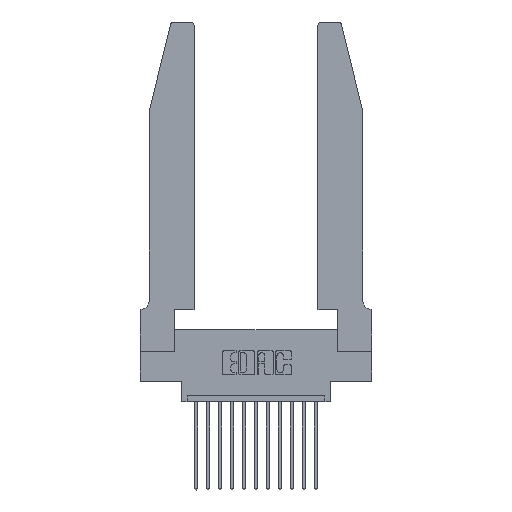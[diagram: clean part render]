
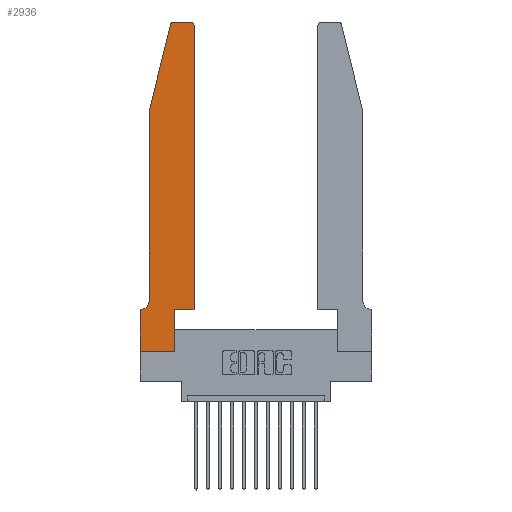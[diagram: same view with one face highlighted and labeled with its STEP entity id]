
A CAD part, top view. The second image highlights one B-rep face of the part: STEP entity #2936.
In plain terms, the highlighted planar face has unit normal (0, 0, 1).
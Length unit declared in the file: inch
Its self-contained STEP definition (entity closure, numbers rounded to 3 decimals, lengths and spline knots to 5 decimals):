
#218 = CARTESIAN_POINT ( 'NONE',  ( 0.4505, 0.35, 0.37 ) ) ;
#524 = VECTOR ( 'NONE', #14686, 39.37008 ) ;
#703 = EDGE_CURVE ( 'NONE', #8851, #9244, #15966, .T. ) ;
#982 = CIRCLE ( 'NONE', #16552, 0.03 ) ;
#1144 = DIRECTION ( 'NONE',  ( 0., 0., -1. ) ) ;
#1153 = VERTEX_POINT ( 'NONE', #10646 ) ;
#1283 = ORIENTED_EDGE ( 'NONE', *, *, #15744, .T. ) ;
#1288 = VERTEX_POINT ( 'NONE', #3385 ) ;
#1454 = VECTOR ( 'NONE', #7306, 39.37008 ) ;
#1493 = AXIS2_PLACEMENT_3D ( 'NONE', #8289, #6906, #9633 ) ;
#1784 = LINE ( 'NONE', #15806, #14376 ) ;
#2375 = DIRECTION ( 'NONE',  ( 0., 0., 1. ) ) ;
#2543 = DIRECTION ( 'NONE',  ( 1., 0., 0. ) ) ;
#2564 = DIRECTION ( 'NONE',  ( -1., 0., 0. ) ) ;
#2749 = CARTESIAN_POINT ( 'NONE',  ( 0., 0., 0.37 ) ) ;
#2924 = ORIENTED_EDGE ( 'NONE', *, *, #3861, .T. ) ;
#2930 = LINE ( 'NONE', #4399, #8323 ) ;
#2936 = ADVANCED_FACE ( 'NONE', ( #8932 ), #13617, .T. ) ;
#3160 = CARTESIAN_POINT ( 'NONE',  ( 0.0055, 0.42, 0.37 ) ) ;
#3186 = LINE ( 'NONE', #16306, #5674 ) ;
#3196 = CARTESIAN_POINT ( 'NONE',  ( 0.25487, 2.72718, 0.37 ) ) ;
#3385 = CARTESIAN_POINT ( 'NONE',  ( 0.4505, 2.72, 0.37 ) ) ;
#3501 = DIRECTION ( 'NONE',  ( 1., 0., 0. ) ) ;
#3754 = EDGE_CURVE ( 'NONE', #15137, #3875, #2930, .T. ) ;
#3861 = EDGE_CURVE ( 'NONE', #1153, #13302, #14398, .T. ) ;
#3875 = VERTEX_POINT ( 'NONE', #11994 ) ;
#4043 = CARTESIAN_POINT ( 'NONE',  ( 0.2865, 0.35, 0.37 ) ) ;
#4224 = VECTOR ( 'NONE', #15004, 39.37008 ) ;
#4336 = CARTESIAN_POINT ( 'NONE',  ( 0.0755, 2., 0.37 ) ) ;
#4377 = CARTESIAN_POINT ( 'NONE',  ( 0.2865, 0., 0.37 ) ) ;
#4399 = CARTESIAN_POINT ( 'NONE',  ( 0.2605, 2.75, 0.37 ) ) ;
#4722 = CARTESIAN_POINT ( 'NONE',  ( 0.0055, 0.35, 0.37 ) ) ;
#5094 = ORIENTED_EDGE ( 'NONE', *, *, #10176, .T. ) ;
#5428 = VECTOR ( 'NONE', #3501, 39.37008 ) ;
#5515 = DIRECTION ( 'NONE',  ( 0., 1., 0. ) ) ;
#5674 = VECTOR ( 'NONE', #5515, 39.37008 ) ;
#5723 = EDGE_CURVE ( 'NONE', #1288, #15137, #982, .T. ) ;
#5820 = CIRCLE ( 'NONE', #13516, 0.07 ) ;
#6085 = CARTESIAN_POINT ( 'NONE',  ( 0.0755, 0.42, 0.37 ) ) ;
#6169 = VERTEX_POINT ( 'NONE', #4722 ) ;
#6243 = VECTOR ( 'NONE', #14465, 39.37008 ) ;
#6330 = CARTESIAN_POINT ( 'NONE',  ( 0.4205, 2.72, 0.37 ) ) ;
#6340 = DIRECTION ( 'NONE',  ( -1., 0., 0. ) ) ;
#6342 = ORIENTED_EDGE ( 'NONE', *, *, #703, .T. ) ;
#6404 = EDGE_CURVE ( 'NONE', #6169, #1153, #1784, .T. ) ;
#6906 = DIRECTION ( 'NONE',  ( 0., 0., 1. ) ) ;
#7190 = VERTEX_POINT ( 'NONE', #8349 ) ;
#7306 = DIRECTION ( 'NONE',  ( 1., 0., 0. ) ) ;
#7482 = CARTESIAN_POINT ( 'NONE',  ( 0., 0., 0.37 ) ) ;
#8289 = CARTESIAN_POINT ( 'NONE',  ( 0., 0.35, 0.37 ) ) ;
#8323 = VECTOR ( 'NONE', #13787, 39.37008 ) ;
#8349 = CARTESIAN_POINT ( 'NONE',  ( 0.0755, 2., 0.37 ) ) ;
#8526 = LINE ( 'NONE', #11234, #14650 ) ;
#8674 = VERTEX_POINT ( 'NONE', #6085 ) ;
#8798 = LINE ( 'NONE', #4336, #4224 ) ;
#8851 = VERTEX_POINT ( 'NONE', #4043 ) ;
#8932 = FACE_OUTER_BOUND ( 'NONE', #9172, .T. ) ;
#9172 = EDGE_LOOP ( 'NONE', ( #11624, #17141, #5094, #13546, #16182, #11566, #2924, #14757, #11115, #6342, #1283, #9913 ) ) ;
#9244 = VERTEX_POINT ( 'NONE', #218 ) ;
#9633 = DIRECTION ( 'NONE',  ( 1., 0., 0. ) ) ;
#9913 = ORIENTED_EDGE ( 'NONE', *, *, #5723, .T. ) ;
#9942 = DIRECTION ( 'NONE',  ( -0.239, -0.971, 0. ) ) ;
#10126 = DIRECTION ( 'NONE',  ( 0., 0., 1. ) ) ;
#10156 = EDGE_CURVE ( 'NONE', #13302, #10535, #10426, .T. ) ;
#10176 = EDGE_CURVE ( 'NONE', #16699, #7190, #8526, .T. ) ;
#10389 = CARTESIAN_POINT ( 'NONE',  ( 0., 0., 0.37 ) ) ;
#10426 = LINE ( 'NONE', #7482, #5428 ) ;
#10501 = EDGE_CURVE ( 'NONE', #8674, #6169, #5820, .T. ) ;
#10535 = VERTEX_POINT ( 'NONE', #4377 ) ;
#10646 = CARTESIAN_POINT ( 'NONE',  ( 0., 0.35, 0.37 ) ) ;
#11016 = CARTESIAN_POINT ( 'NONE',  ( 0.4205, 2.75, 0.37 ) ) ;
#11039 = EDGE_CURVE ( 'NONE', #10535, #8851, #11254, .T. ) ;
#11115 = ORIENTED_EDGE ( 'NONE', *, *, #11039, .T. ) ;
#11234 = CARTESIAN_POINT ( 'NONE',  ( 0.0755, 2., 0.37 ) ) ;
#11254 = LINE ( 'NONE', #11705, #6243 ) ;
#11566 = ORIENTED_EDGE ( 'NONE', *, *, #6404, .T. ) ;
#11624 = ORIENTED_EDGE ( 'NONE', *, *, #3754, .T. ) ;
#11705 = CARTESIAN_POINT ( 'NONE',  ( 0.2865, 0.35, 0.37 ) ) ;
#11856 = CIRCLE ( 'NONE', #16314, 0.03 ) ;
#11994 = CARTESIAN_POINT ( 'NONE',  ( 0.284, 2.75, 0.37 ) ) ;
#12715 = EDGE_CURVE ( 'NONE', #3875, #16699, #11856, .T. ) ;
#13302 = VERTEX_POINT ( 'NONE', #10389 ) ;
#13516 = AXIS2_PLACEMENT_3D ( 'NONE', #3160, #1144, #2564 ) ;
#13546 = ORIENTED_EDGE ( 'NONE', *, *, #15742, .T. ) ;
#13617 = PLANE ( 'NONE',  #1493 ) ;
#13787 = DIRECTION ( 'NONE',  ( -1., 0., 0. ) ) ;
#14376 = VECTOR ( 'NONE', #6340, 39.37008 ) ;
#14398 = LINE ( 'NONE', #2749, #524 ) ;
#14465 = DIRECTION ( 'NONE',  ( 0., 1., 0. ) ) ;
#14650 = VECTOR ( 'NONE', #9942, 39.37008 ) ;
#14686 = DIRECTION ( 'NONE',  ( 0., -1., 0. ) ) ;
#14757 = ORIENTED_EDGE ( 'NONE', *, *, #10156, .T. ) ;
#15004 = DIRECTION ( 'NONE',  ( 0., -1., 0. ) ) ;
#15137 = VERTEX_POINT ( 'NONE', #11016 ) ;
#15338 = CARTESIAN_POINT ( 'NONE',  ( 0.4505, 0.35, 0.37 ) ) ;
#15623 = CARTESIAN_POINT ( 'NONE',  ( 0.284, 2.72, 0.37 ) ) ;
#15742 = EDGE_CURVE ( 'NONE', #7190, #8674, #8798, .T. ) ;
#15744 = EDGE_CURVE ( 'NONE', #9244, #1288, #3186, .T. ) ;
#15806 = CARTESIAN_POINT ( 'NONE',  ( 0.0755, 0.35, 0.37 ) ) ;
#15966 = LINE ( 'NONE', #15338, #1454 ) ;
#16182 = ORIENTED_EDGE ( 'NONE', *, *, #10501, .T. ) ;
#16306 = CARTESIAN_POINT ( 'NONE',  ( 0.4505, 0.35, 0.37 ) ) ;
#16314 = AXIS2_PLACEMENT_3D ( 'NONE', #15623, #10126, #16918 ) ;
#16552 = AXIS2_PLACEMENT_3D ( 'NONE', #6330, #2375, #2543 ) ;
#16699 = VERTEX_POINT ( 'NONE', #3196 ) ;
#16918 = DIRECTION ( 'NONE',  ( 1., 0., 0. ) ) ;
#17141 = ORIENTED_EDGE ( 'NONE', *, *, #12715, .T. ) ;
